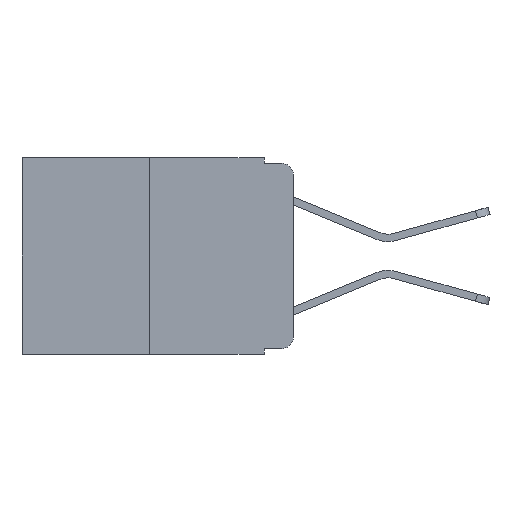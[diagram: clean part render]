
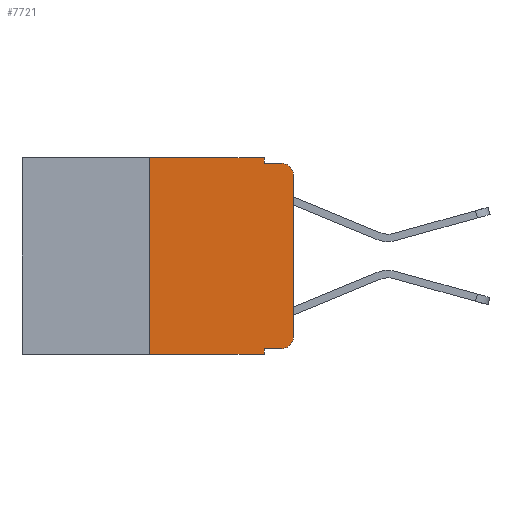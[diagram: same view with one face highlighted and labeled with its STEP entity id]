
A CAD part, left-side view. The second image highlights one B-rep face of the part: STEP entity #7721.
In plain terms, the highlighted planar face has unit normal (-1, 0, 0).
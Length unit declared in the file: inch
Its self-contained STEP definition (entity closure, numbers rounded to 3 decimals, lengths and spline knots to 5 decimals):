
#29 = DIRECTION ( 'NONE',  ( 0., 0., 1. ) ) ;
#33 = VECTOR ( 'NONE', #29, 39.37008 ) ;
#90 = EDGE_CURVE ( 'NONE', #11160, #312, #9824, .T. ) ;
#96 = VERTEX_POINT ( 'NONE', #3077 ) ;
#97 = CARTESIAN_POINT ( 'NONE',  ( 0., 0.02, -0.01 ) ) ;
#312 = VERTEX_POINT ( 'NONE', #10073 ) ;
#741 = EDGE_CURVE ( 'NONE', #96, #11160, #11455, .T. ) ;
#1103 = DIRECTION ( 'NONE',  ( 0., 0., -1. ) ) ;
#1368 = DIRECTION ( 'NONE',  ( -1., 0., 0. ) ) ;
#1377 = VERTEX_POINT ( 'NONE', #11120 ) ;
#1453 = PLANE ( 'NONE',  #4760 ) ;
#1515 = DIRECTION ( 'NONE',  ( 0., 0., -1. ) ) ;
#1850 = DIRECTION ( 'NONE',  ( 0., -1., 0. ) ) ;
#1876 = AXIS2_PLACEMENT_3D ( 'NONE', #10446, #5326, #1103 ) ;
#1899 = LINE ( 'NONE', #9317, #6725 ) ;
#1933 = ORIENTED_EDGE ( 'NONE', *, *, #4531, .F. ) ;
#2059 = EDGE_CURVE ( 'NONE', #96, #2249, #1899, .T. ) ;
#2169 = CARTESIAN_POINT ( 'NONE',  ( 0., 0., -0.03 ) ) ;
#2249 = VERTEX_POINT ( 'NONE', #7311 ) ;
#2369 = EDGE_CURVE ( 'NONE', #7520, #9536, #8065, .T. ) ;
#2394 = DIRECTION ( 'NONE',  ( 1., 0., 0. ) ) ;
#2426 = CARTESIAN_POINT ( 'NONE',  ( 0., 0.051, 0. ) ) ;
#2503 = ORIENTED_EDGE ( 'NONE', *, *, #741, .T. ) ;
#2547 = VECTOR ( 'NONE', #1850, 39.37008 ) ;
#2599 = DIRECTION ( 'NONE',  ( 0., 0., 1. ) ) ;
#2661 = EDGE_CURVE ( 'NONE', #2847, #7520, #9926, .T. ) ;
#2756 = VERTEX_POINT ( 'NONE', #2169 ) ;
#2847 = VERTEX_POINT ( 'NONE', #4702 ) ;
#2944 = VECTOR ( 'NONE', #2599, 39.37008 ) ;
#3077 = CARTESIAN_POINT ( 'NONE',  ( 0., 0.051, -0.333 ) ) ;
#3146 = FACE_OUTER_BOUND ( 'NONE', #9157, .T. ) ;
#3277 = EDGE_CURVE ( 'NONE', #9536, #1377, #9166, .T. ) ;
#3429 = CARTESIAN_POINT ( 'NONE',  ( 0., 0.02, -0.313 ) ) ;
#3842 = CIRCLE ( 'NONE', #1876, 0.02 ) ;
#4109 = ORIENTED_EDGE ( 'NONE', *, *, #5769, .T. ) ;
#4498 = CARTESIAN_POINT ( 'NONE',  ( 0., 0.25, 0. ) ) ;
#4531 = EDGE_CURVE ( 'NONE', #1377, #11375, #5022, .T. ) ;
#4702 = CARTESIAN_POINT ( 'NONE',  ( 0., 0.25, -0.343 ) ) ;
#4760 = AXIS2_PLACEMENT_3D ( 'NONE', #7759, #2394, #8663 ) ;
#4972 = ORIENTED_EDGE ( 'NONE', *, *, #90, .T. ) ;
#5022 = LINE ( 'NONE', #6401, #2547 ) ;
#5044 = CARTESIAN_POINT ( 'NONE',  ( 0., 0.473, -0.343 ) ) ;
#5145 = EDGE_CURVE ( 'NONE', #2756, #11375, #3842, .T. ) ;
#5326 = DIRECTION ( 'NONE',  ( -1., 0., 0. ) ) ;
#5414 = LINE ( 'NONE', #7933, #2944 ) ;
#5769 = EDGE_CURVE ( 'NONE', #312, #2756, #5414, .T. ) ;
#5956 = DIRECTION ( 'NONE',  ( 0., -1., 0. ) ) ;
#6171 = DIRECTION ( 'NONE',  ( 0., 0., -1. ) ) ;
#6289 = CARTESIAN_POINT ( 'NONE',  ( 0., 0.051, -0.333 ) ) ;
#6401 = CARTESIAN_POINT ( 'NONE',  ( 0., 0.051, -0.01 ) ) ;
#6422 = VECTOR ( 'NONE', #5956, 39.37008 ) ;
#6725 = VECTOR ( 'NONE', #9283, 39.37008 ) ;
#6749 = ORIENTED_EDGE ( 'NONE', *, *, #3277, .F. ) ;
#6824 = VECTOR ( 'NONE', #1515, 39.37008 ) ;
#6845 = AXIS2_PLACEMENT_3D ( 'NONE', #3429, #1368, #6171 ) ;
#6869 = DIRECTION ( 'NONE',  ( 0., -1., 0. ) ) ;
#6882 = CARTESIAN_POINT ( 'NONE',  ( 0., 0.473, 0. ) ) ;
#7014 = ORIENTED_EDGE ( 'NONE', *, *, #9571, .T. ) ;
#7087 = CARTESIAN_POINT ( 'NONE',  ( 0., 0.25, 0. ) ) ;
#7311 = CARTESIAN_POINT ( 'NONE',  ( 0., 0.051, -0.343 ) ) ;
#7520 = VERTEX_POINT ( 'NONE', #7087 ) ;
#7721 = ADVANCED_FACE ( 'NONE', ( #3146 ), #1453, .F. ) ;
#7759 = CARTESIAN_POINT ( 'NONE',  ( 0., 0.473, 0. ) ) ;
#7933 = CARTESIAN_POINT ( 'NONE',  ( 0., 0., 0. ) ) ;
#8065 = LINE ( 'NONE', #6882, #10068 ) ;
#8397 = DIRECTION ( 'NONE',  ( 0., -1., 0. ) ) ;
#8663 = DIRECTION ( 'NONE',  ( 0., 0., -1. ) ) ;
#9080 = ORIENTED_EDGE ( 'NONE', *, *, #2369, .F. ) ;
#9157 = EDGE_LOOP ( 'NONE', ( #4109, #10970, #1933, #6749, #9080, #11215, #7014, #9347, #2503, #4972 ) ) ;
#9166 = LINE ( 'NONE', #2426, #6824 ) ;
#9283 = DIRECTION ( 'NONE',  ( 0., 0., -1. ) ) ;
#9317 = CARTESIAN_POINT ( 'NONE',  ( 0., 0.051, 0. ) ) ;
#9330 = VECTOR ( 'NONE', #8397, 39.37008 ) ;
#9347 = ORIENTED_EDGE ( 'NONE', *, *, #2059, .F. ) ;
#9536 = VERTEX_POINT ( 'NONE', #10162 ) ;
#9571 = EDGE_CURVE ( 'NONE', #2847, #2249, #11156, .T. ) ;
#9824 = CIRCLE ( 'NONE', #6845, 0.02 ) ;
#9926 = LINE ( 'NONE', #4498, #33 ) ;
#10068 = VECTOR ( 'NONE', #6869, 39.37008 ) ;
#10073 = CARTESIAN_POINT ( 'NONE',  ( 0., 0., -0.313 ) ) ;
#10162 = CARTESIAN_POINT ( 'NONE',  ( 0., 0.051, 0. ) ) ;
#10370 = CARTESIAN_POINT ( 'NONE',  ( 0., 0.02, -0.333 ) ) ;
#10446 = CARTESIAN_POINT ( 'NONE',  ( 0., 0.02, -0.03 ) ) ;
#10970 = ORIENTED_EDGE ( 'NONE', *, *, #5145, .T. ) ;
#11120 = CARTESIAN_POINT ( 'NONE',  ( 0., 0.051, -0.01 ) ) ;
#11156 = LINE ( 'NONE', #5044, #6422 ) ;
#11160 = VERTEX_POINT ( 'NONE', #10370 ) ;
#11215 = ORIENTED_EDGE ( 'NONE', *, *, #2661, .F. ) ;
#11375 = VERTEX_POINT ( 'NONE', #97 ) ;
#11455 = LINE ( 'NONE', #6289, #9330 ) ;
